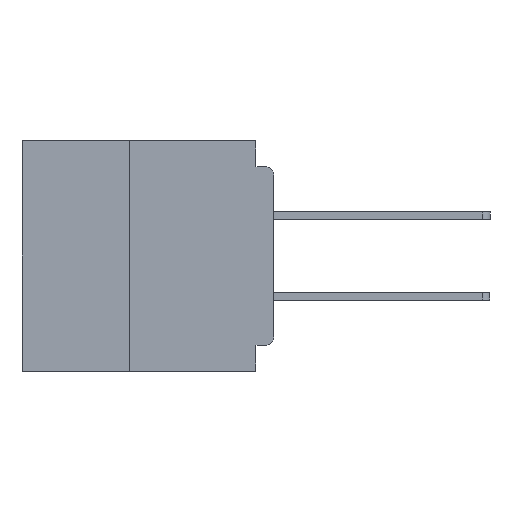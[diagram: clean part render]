
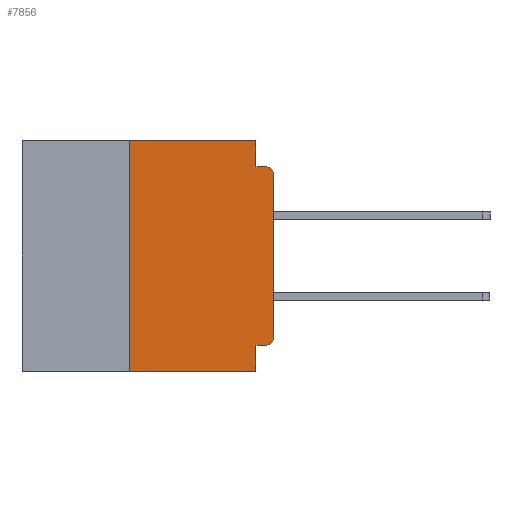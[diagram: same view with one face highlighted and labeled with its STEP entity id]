
A CAD part, left-side view. The second image highlights one B-rep face of the part: STEP entity #7856.
In plain terms, the highlighted planar face has unit normal (-1, 0, 0).
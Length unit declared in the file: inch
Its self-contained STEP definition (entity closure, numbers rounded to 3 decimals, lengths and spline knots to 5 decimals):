
#649 = ORIENTED_EDGE ( 'NONE', *, *, #51181, .T. ) ;
#1757 = ORIENTED_EDGE ( 'NONE', *, *, #43339, .F. ) ;
#2133 = VERTEX_POINT ( 'NONE', #22228 ) ;
#2396 = DIRECTION ( 'NONE',  ( 0., -1., 0. ) ) ;
#2973 = DIRECTION ( 'NONE',  ( 0., 0., -1. ) ) ;
#4004 = EDGE_CURVE ( 'NONE', #48940, #9835, #46480, .T. ) ;
#4314 = ORIENTED_EDGE ( 'NONE', *, *, #18977, .F. ) ;
#4733 = CARTESIAN_POINT ( 'NONE',  ( 0., 0.437, 0. ) ) ;
#4926 = VECTOR ( 'NONE', #22101, 39.37008 ) ;
#5278 = CARTESIAN_POINT ( 'NONE',  ( 0., 0.031, -0.4 ) ) ;
#5684 = CARTESIAN_POINT ( 'NONE',  ( 0., 0.015, -0.34 ) ) ;
#5804 = CARTESIAN_POINT ( 'NONE',  ( 0., 0.25, 0. ) ) ;
#5933 = DIRECTION ( 'NONE',  ( 0., 0., -1. ) ) ;
#6108 = ORIENTED_EDGE ( 'NONE', *, *, #41915, .F. ) ;
#7218 = DIRECTION ( 'NONE',  ( 0., 0., 1. ) ) ;
#7454 = CARTESIAN_POINT ( 'NONE',  ( 0., 0.031, 0. ) ) ;
#7856 = ADVANCED_FACE ( 'NONE', ( #12180 ), #26053, .F. ) ;
#9759 = DIRECTION ( 'NONE',  ( 0., 0., -1. ) ) ;
#9835 = VERTEX_POINT ( 'NONE', #15939 ) ;
#10156 = LINE ( 'NONE', #7454, #30304 ) ;
#11950 = AXIS2_PLACEMENT_3D ( 'NONE', #41953, #30074, #5933 ) ;
#11954 = CARTESIAN_POINT ( 'NONE',  ( 0., 0.25, -0.4 ) ) ;
#11960 = VECTOR ( 'NONE', #37498, 39.37008 ) ;
#12180 = FACE_OUTER_BOUND ( 'NONE', #23607, .T. ) ;
#12941 = ORIENTED_EDGE ( 'NONE', *, *, #44594, .F. ) ;
#13223 = VECTOR ( 'NONE', #2396, 39.37008 ) ;
#14169 = VERTEX_POINT ( 'NONE', #43116 ) ;
#15074 = CARTESIAN_POINT ( 'NONE',  ( 0., 0., -0.355 ) ) ;
#15939 = CARTESIAN_POINT ( 'NONE',  ( 0., 0.031, -0.4 ) ) ;
#17106 = EDGE_CURVE ( 'NONE', #27148, #39692, #44198, .T. ) ;
#17874 = CARTESIAN_POINT ( 'NONE',  ( 0., 0.031, -0.045 ) ) ;
#18073 = VECTOR ( 'NONE', #48943, 39.37008 ) ;
#18698 = ORIENTED_EDGE ( 'NONE', *, *, #4004, .T. ) ;
#18977 = EDGE_CURVE ( 'NONE', #29580, #50892, #10156, .T. ) ;
#19322 = LINE ( 'NONE', #4733, #18073 ) ;
#22087 = AXIS2_PLACEMENT_3D ( 'NONE', #51041, #27185, #2973 ) ;
#22101 = DIRECTION ( 'NONE',  ( 0., -1., 0. ) ) ;
#22228 = CARTESIAN_POINT ( 'NONE',  ( 0., 0., -0.34 ) ) ;
#23607 = EDGE_LOOP ( 'NONE', ( #649, #47619, #1757, #4314, #12941, #50292, #18698, #6108, #30833, #49692 ) ) ;
#23977 = LINE ( 'NONE', #5278, #11960 ) ;
#24863 = VECTOR ( 'NONE', #7218, 39.37008 ) ;
#26053 = PLANE ( 'NONE',  #11950 ) ;
#26153 = CARTESIAN_POINT ( 'NONE',  ( 0., 0., -0.045 ) ) ;
#26584 = CARTESIAN_POINT ( 'NONE',  ( 0., 0.437, -0.4 ) ) ;
#26667 = CARTESIAN_POINT ( 'NONE',  ( 0., 0.25, -0.4 ) ) ;
#27148 = VERTEX_POINT ( 'NONE', #32078 ) ;
#27185 = DIRECTION ( 'NONE',  ( -1., 0., 0. ) ) ;
#29573 = EDGE_CURVE ( 'NONE', #48940, #42010, #35521, .T. ) ;
#29580 = VERTEX_POINT ( 'NONE', #43373 ) ;
#29733 = VECTOR ( 'NONE', #39777, 39.37008 ) ;
#29876 = CARTESIAN_POINT ( 'NONE',  ( 0., 0.015, -0.045 ) ) ;
#30074 = DIRECTION ( 'NONE',  ( 1., 0., 0. ) ) ;
#30304 = VECTOR ( 'NONE', #39619, 39.37008 ) ;
#30833 = ORIENTED_EDGE ( 'NONE', *, *, #32013, .F. ) ;
#30939 = CARTESIAN_POINT ( 'NONE',  ( 0., 0.015, -0.355 ) ) ;
#32013 = EDGE_CURVE ( 'NONE', #34643, #14169, #43974, .T. ) ;
#32078 = CARTESIAN_POINT ( 'NONE',  ( 0., 0., -0.06 ) ) ;
#33874 = DIRECTION ( 'NONE',  ( -1., 0., 0. ) ) ;
#34643 = VERTEX_POINT ( 'NONE', #30939 ) ;
#35521 = LINE ( 'NONE', #11954, #24863 ) ;
#35771 = CARTESIAN_POINT ( 'NONE',  ( 0., 0., 0. ) ) ;
#37062 = LINE ( 'NONE', #26153, #4926 ) ;
#37498 = DIRECTION ( 'NONE',  ( 0., 0., -1. ) ) ;
#39554 = CIRCLE ( 'NONE', #50069, 0.015 ) ;
#39619 = DIRECTION ( 'NONE',  ( 0., 0., -1. ) ) ;
#39692 = VERTEX_POINT ( 'NONE', #29876 ) ;
#39777 = DIRECTION ( 'NONE',  ( 0., 0., 1. ) ) ;
#41915 = EDGE_CURVE ( 'NONE', #14169, #9835, #23977, .T. ) ;
#41953 = CARTESIAN_POINT ( 'NONE',  ( 0., 0.437, 0. ) ) ;
#42010 = VERTEX_POINT ( 'NONE', #5804 ) ;
#43116 = CARTESIAN_POINT ( 'NONE',  ( 0., 0.031, -0.355 ) ) ;
#43138 = DIRECTION ( 'NONE',  ( 0., 1., 0. ) ) ;
#43274 = EDGE_CURVE ( 'NONE', #34643, #2133, #39554, .T. ) ;
#43339 = EDGE_CURVE ( 'NONE', #50892, #39692, #37062, .T. ) ;
#43373 = CARTESIAN_POINT ( 'NONE',  ( 0., 0.031, 0. ) ) ;
#43974 = LINE ( 'NONE', #15074, #45228 ) ;
#44198 = CIRCLE ( 'NONE', #22087, 0.015 ) ;
#44594 = EDGE_CURVE ( 'NONE', #42010, #29580, #19322, .T. ) ;
#45228 = VECTOR ( 'NONE', #43138, 39.37008 ) ;
#46480 = LINE ( 'NONE', #26584, #13223 ) ;
#47619 = ORIENTED_EDGE ( 'NONE', *, *, #17106, .T. ) ;
#48940 = VERTEX_POINT ( 'NONE', #26667 ) ;
#48943 = DIRECTION ( 'NONE',  ( 0., -1., 0. ) ) ;
#49692 = ORIENTED_EDGE ( 'NONE', *, *, #43274, .T. ) ;
#50069 = AXIS2_PLACEMENT_3D ( 'NONE', #5684, #33874, #9759 ) ;
#50292 = ORIENTED_EDGE ( 'NONE', *, *, #29573, .F. ) ;
#50892 = VERTEX_POINT ( 'NONE', #17874 ) ;
#50931 = LINE ( 'NONE', #35771, #29733 ) ;
#51041 = CARTESIAN_POINT ( 'NONE',  ( 0., 0.015, -0.06 ) ) ;
#51181 = EDGE_CURVE ( 'NONE', #2133, #27148, #50931, .T. ) ;
